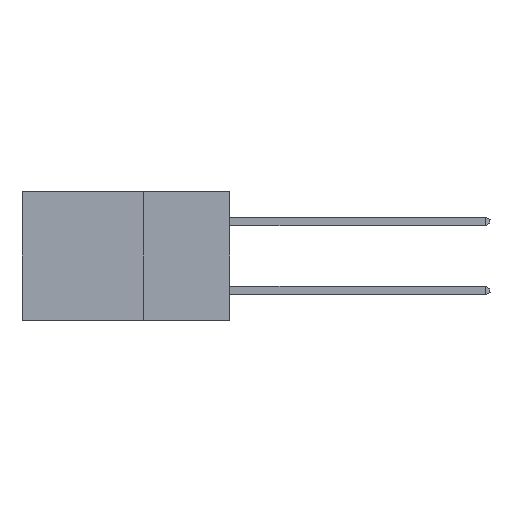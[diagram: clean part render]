
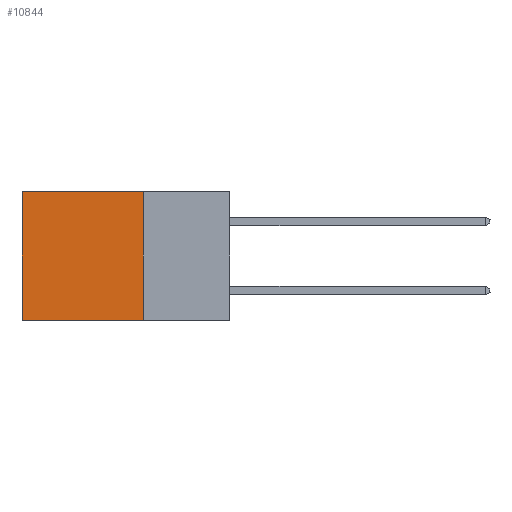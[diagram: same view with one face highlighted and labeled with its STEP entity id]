
A CAD part, left-side view. The second image highlights one B-rep face of the part: STEP entity #10844.
In plain terms, the highlighted planar face has unit normal (-1, 0, 0).
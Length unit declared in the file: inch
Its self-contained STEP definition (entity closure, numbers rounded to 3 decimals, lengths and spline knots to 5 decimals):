
#596 = CARTESIAN_POINT ( 'NONE',  ( 0.298, 0.25, 0. ) ) ;
#1520 = CARTESIAN_POINT ( 'NONE',  ( 0.298, 0.6, -0.37 ) ) ;
#1639 = FACE_OUTER_BOUND ( 'NONE', #32032, .T. ) ;
#2302 = CARTESIAN_POINT ( 'NONE',  ( 0.298, 0.25, -0.37 ) ) ;
#3138 = CARTESIAN_POINT ( 'NONE',  ( 0.298, 0.6, 0. ) ) ;
#4104 = ORIENTED_EDGE ( 'NONE', *, *, #14840, .F. ) ;
#4233 = ORIENTED_EDGE ( 'NONE', *, *, #22059, .F. ) ;
#4339 = CARTESIAN_POINT ( 'NONE',  ( 0.298, 0.25, 0. ) ) ;
#4442 = LINE ( 'NONE', #2302, #26721 ) ;
#4677 = VERTEX_POINT ( 'NONE', #8043 ) ;
#4988 = LINE ( 'NONE', #4339, #31239 ) ;
#8043 = CARTESIAN_POINT ( 'NONE',  ( 0.298, 0.25, 0. ) ) ;
#9359 = CARTESIAN_POINT ( 'NONE',  ( 0.298, 0.25, 0. ) ) ;
#10844 = ADVANCED_FACE ( 'NONE', ( #1639 ), #11626, .F. ) ;
#11090 = CARTESIAN_POINT ( 'NONE',  ( 0.298, 0.6, 0. ) ) ;
#11626 = PLANE ( 'NONE',  #22625 ) ;
#14306 = DIRECTION ( 'NONE',  ( 1., 0., 0. ) ) ;
#14349 = EDGE_CURVE ( 'NONE', #14398, #28120, #18656, .T. ) ;
#14398 = VERTEX_POINT ( 'NONE', #11090 ) ;
#14616 = DIRECTION ( 'NONE',  ( 0., 0., -1. ) ) ;
#14840 = EDGE_CURVE ( 'NONE', #29964, #28120, #4442, .T. ) ;
#15885 = VECTOR ( 'NONE', #22627, 39.37008 ) ;
#18631 = DIRECTION ( 'NONE',  ( 0., 1., 0. ) ) ;
#18656 = LINE ( 'NONE', #3138, #15885 ) ;
#19595 = ORIENTED_EDGE ( 'NONE', *, *, #14349, .T. ) ;
#19988 = LINE ( 'NONE', #596, #25182 ) ;
#22059 = EDGE_CURVE ( 'NONE', #4677, #29964, #4988, .T. ) ;
#22575 = ORIENTED_EDGE ( 'NONE', *, *, #23699, .T. ) ;
#22625 = AXIS2_PLACEMENT_3D ( 'NONE', #9359, #14306, #24208 ) ;
#22627 = DIRECTION ( 'NONE',  ( 0., 0., -1. ) ) ;
#23699 = EDGE_CURVE ( 'NONE', #4677, #14398, #19988, .T. ) ;
#24208 = DIRECTION ( 'NONE',  ( 0., 0., -1. ) ) ;
#25182 = VECTOR ( 'NONE', #18631, 39.37008 ) ;
#26721 = VECTOR ( 'NONE', #32643, 39.37008 ) ;
#28059 = CARTESIAN_POINT ( 'NONE',  ( 0.298, 0.25, -0.37 ) ) ;
#28120 = VERTEX_POINT ( 'NONE', #1520 ) ;
#29964 = VERTEX_POINT ( 'NONE', #28059 ) ;
#31239 = VECTOR ( 'NONE', #14616, 39.37008 ) ;
#32032 = EDGE_LOOP ( 'NONE', ( #19595, #4104, #4233, #22575 ) ) ;
#32643 = DIRECTION ( 'NONE',  ( 0., 1., 0. ) ) ;
